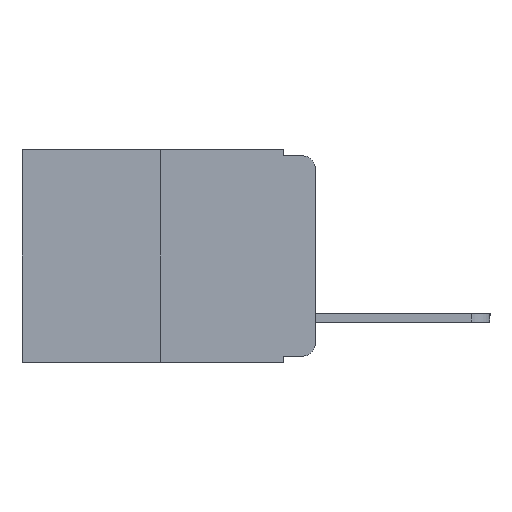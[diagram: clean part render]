
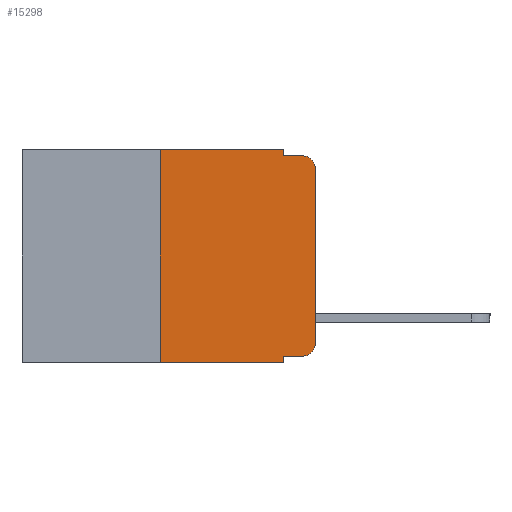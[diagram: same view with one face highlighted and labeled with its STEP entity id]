
A CAD part, left-side view. The second image highlights one B-rep face of the part: STEP entity #15298.
In plain terms, the highlighted planar face has unit normal (-1, 0, 0).
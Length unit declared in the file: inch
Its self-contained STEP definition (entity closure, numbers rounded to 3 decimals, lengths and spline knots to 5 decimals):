
#88 = ORIENTED_EDGE ( 'NONE', *, *, #817, .T. ) ;
#279 = ORIENTED_EDGE ( 'NONE', *, *, #12013, .T. ) ;
#771 = FACE_OUTER_BOUND ( 'NONE', #18721, .T. ) ;
#817 = EDGE_CURVE ( 'NONE', #15116, #7499, #22352, .T. ) ;
#1057 = AXIS2_PLACEMENT_3D ( 'NONE', #5909, #19094, #7831 ) ;
#1493 = CARTESIAN_POINT ( 'NONE',  ( 0., 0.051, 0. ) ) ;
#1523 = VECTOR ( 'NONE', #21188, 39.37008 ) ;
#1638 = DIRECTION ( 'NONE',  ( -1., 0., 0. ) ) ;
#2281 = ORIENTED_EDGE ( 'NONE', *, *, #14551, .T. ) ;
#2442 = CARTESIAN_POINT ( 'NONE',  ( 0., 0.02, -0.333 ) ) ;
#2536 = CIRCLE ( 'NONE', #8061, 0.02 ) ;
#2615 = LINE ( 'NONE', #15523, #22114 ) ;
#3060 = EDGE_CURVE ( 'NONE', #20152, #16108, #15044, .T. ) ;
#3499 = DIRECTION ( 'NONE',  ( 0., 0., 1. ) ) ;
#3698 = CARTESIAN_POINT ( 'NONE',  ( 0., 0.02, -0.01 ) ) ;
#4322 = EDGE_CURVE ( 'NONE', #4504, #20152, #10887, .T. ) ;
#4443 = CARTESIAN_POINT ( 'NONE',  ( 0., 0.051, -0.01 ) ) ;
#4504 = VERTEX_POINT ( 'NONE', #13933 ) ;
#5098 = LINE ( 'NONE', #5103, #19557 ) ;
#5103 = CARTESIAN_POINT ( 'NONE',  ( 0., 0.25, 0. ) ) ;
#5539 = VERTEX_POINT ( 'NONE', #3698 ) ;
#5615 = EDGE_CURVE ( 'NONE', #4504, #7499, #20191, .T. ) ;
#5731 = VECTOR ( 'NONE', #13542, 39.37008 ) ;
#5909 = CARTESIAN_POINT ( 'NONE',  ( 0., 0.473, 0. ) ) ;
#5964 = LINE ( 'NONE', #7144, #15464 ) ;
#6265 = EDGE_CURVE ( 'NONE', #24139, #10532, #7795, .T. ) ;
#7144 = CARTESIAN_POINT ( 'NONE',  ( 0., 0.051, 0. ) ) ;
#7226 = DIRECTION ( 'NONE',  ( 0., 0., -1. ) ) ;
#7291 = ORIENTED_EDGE ( 'NONE', *, *, #4322, .T. ) ;
#7499 = VERTEX_POINT ( 'NONE', #23568 ) ;
#7795 = LINE ( 'NONE', #9935, #1523 ) ;
#7831 = DIRECTION ( 'NONE',  ( 0., 0., -1. ) ) ;
#8061 = AXIS2_PLACEMENT_3D ( 'NONE', #8279, #21415, #10174 ) ;
#8188 = EDGE_CURVE ( 'NONE', #15116, #24139, #5098, .T. ) ;
#8279 = CARTESIAN_POINT ( 'NONE',  ( 0., 0.02, -0.03 ) ) ;
#9173 = ORIENTED_EDGE ( 'NONE', *, *, #5615, .F. ) ;
#9448 = EDGE_CURVE ( 'NONE', #10532, #18854, #5964, .T. ) ;
#9526 = DIRECTION ( 'NONE',  ( 0., -1., 0. ) ) ;
#9935 = CARTESIAN_POINT ( 'NONE',  ( 0., 0.473, 0. ) ) ;
#10043 = ORIENTED_EDGE ( 'NONE', *, *, #3060, .T. ) ;
#10174 = DIRECTION ( 'NONE',  ( 0., 0., -1. ) ) ;
#10532 = VERTEX_POINT ( 'NONE', #1493 ) ;
#10757 = EDGE_CURVE ( 'NONE', #18854, #5539, #2615, .T. ) ;
#10887 = LINE ( 'NONE', #11443, #20257 ) ;
#11422 = CARTESIAN_POINT ( 'NONE',  ( 0., 0.25, 0. ) ) ;
#11443 = CARTESIAN_POINT ( 'NONE',  ( 0., 0.051, -0.333 ) ) ;
#11928 = ORIENTED_EDGE ( 'NONE', *, *, #10757, .F. ) ;
#12013 = EDGE_CURVE ( 'NONE', #22676, #5539, #2536, .T. ) ;
#13071 = CARTESIAN_POINT ( 'NONE',  ( 0., 0.02, -0.313 ) ) ;
#13073 = VECTOR ( 'NONE', #3499, 39.37008 ) ;
#13542 = DIRECTION ( 'NONE',  ( 0., 0., -1. ) ) ;
#13933 = CARTESIAN_POINT ( 'NONE',  ( 0., 0.051, -0.333 ) ) ;
#14551 = EDGE_CURVE ( 'NONE', #16108, #22676, #18049, .T. ) ;
#14629 = DIRECTION ( 'NONE',  ( 0., -1., 0. ) ) ;
#14946 = DIRECTION ( 'NONE',  ( 0., 0., -1. ) ) ;
#15044 = CIRCLE ( 'NONE', #20507, 0.02 ) ;
#15116 = VERTEX_POINT ( 'NONE', #20421 ) ;
#15298 = ADVANCED_FACE ( 'NONE', ( #771 ), #15360, .F. ) ;
#15360 = PLANE ( 'NONE',  #1057 ) ;
#15464 = VECTOR ( 'NONE', #7226, 39.37008 ) ;
#15523 = CARTESIAN_POINT ( 'NONE',  ( 0., 0.051, -0.01 ) ) ;
#15587 = ORIENTED_EDGE ( 'NONE', *, *, #6265, .F. ) ;
#16108 = VERTEX_POINT ( 'NONE', #18471 ) ;
#16799 = CARTESIAN_POINT ( 'NONE',  ( 0., 0., 0. ) ) ;
#17409 = DIRECTION ( 'NONE',  ( 0., -1., 0. ) ) ;
#17412 = VECTOR ( 'NONE', #14629, 39.37008 ) ;
#18049 = LINE ( 'NONE', #16799, #13073 ) ;
#18148 = ORIENTED_EDGE ( 'NONE', *, *, #9448, .F. ) ;
#18471 = CARTESIAN_POINT ( 'NONE',  ( 0., 0., -0.313 ) ) ;
#18721 = EDGE_LOOP ( 'NONE', ( #2281, #279, #11928, #18148, #15587, #21678, #88, #9173, #7291, #10043 ) ) ;
#18854 = VERTEX_POINT ( 'NONE', #4443 ) ;
#19094 = DIRECTION ( 'NONE',  ( 1., 0., 0. ) ) ;
#19557 = VECTOR ( 'NONE', #22006, 39.37008 ) ;
#20152 = VERTEX_POINT ( 'NONE', #2442 ) ;
#20191 = LINE ( 'NONE', #22825, #5731 ) ;
#20257 = VECTOR ( 'NONE', #9526, 39.37008 ) ;
#20421 = CARTESIAN_POINT ( 'NONE',  ( 0., 0.25, -0.343 ) ) ;
#20507 = AXIS2_PLACEMENT_3D ( 'NONE', #13071, #1638, #14946 ) ;
#21188 = DIRECTION ( 'NONE',  ( 0., -1., 0. ) ) ;
#21415 = DIRECTION ( 'NONE',  ( -1., 0., 0. ) ) ;
#21678 = ORIENTED_EDGE ( 'NONE', *, *, #8188, .F. ) ;
#22006 = DIRECTION ( 'NONE',  ( 0., 0., 1. ) ) ;
#22114 = VECTOR ( 'NONE', #17409, 39.37008 ) ;
#22352 = LINE ( 'NONE', #23900, #17412 ) ;
#22676 = VERTEX_POINT ( 'NONE', #23521 ) ;
#22825 = CARTESIAN_POINT ( 'NONE',  ( 0., 0.051, 0. ) ) ;
#23521 = CARTESIAN_POINT ( 'NONE',  ( 0., 0., -0.03 ) ) ;
#23568 = CARTESIAN_POINT ( 'NONE',  ( 0., 0.051, -0.343 ) ) ;
#23900 = CARTESIAN_POINT ( 'NONE',  ( 0., 0.473, -0.343 ) ) ;
#24139 = VERTEX_POINT ( 'NONE', #11422 ) ;
